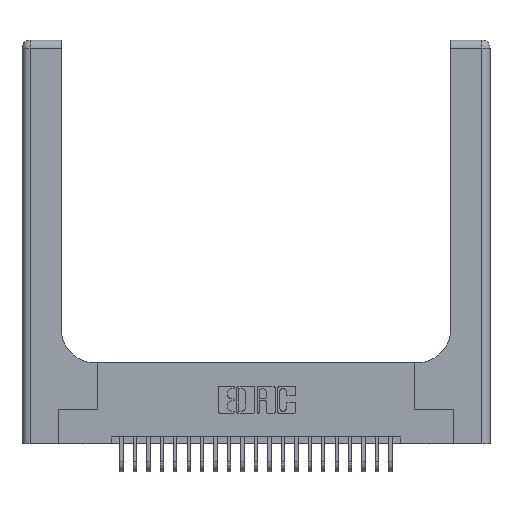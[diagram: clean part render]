
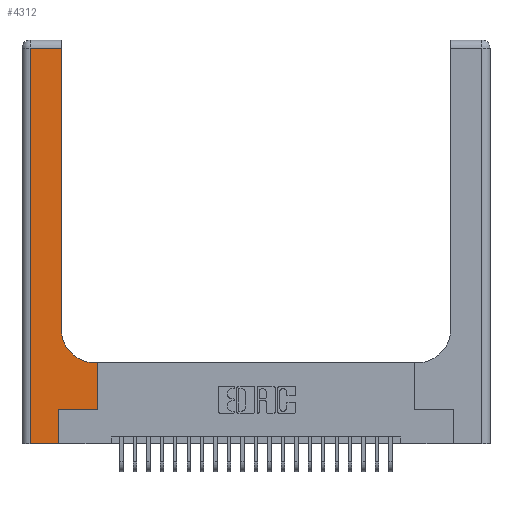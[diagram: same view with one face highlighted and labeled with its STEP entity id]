
A CAD part, top view. The second image highlights one B-rep face of the part: STEP entity #4312.
In plain terms, the highlighted planar face has unit normal (0, 0, 1).
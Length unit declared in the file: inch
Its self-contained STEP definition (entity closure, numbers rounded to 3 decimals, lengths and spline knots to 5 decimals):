
#283 = EDGE_CURVE ( 'NONE', #5069, #25096, #24114, .T. ) ;
#323 = EDGE_CURVE ( 'NONE', #25096, #14885, #16955, .T. ) ;
#327 = EDGE_CURVE ( 'NONE', #7880, #5069, #632, .T. ) ;
#428 = PLANE ( 'NONE',  #16071 ) ;
#632 = LINE ( 'NONE', #15826, #6159 ) ;
#633 = VECTOR ( 'NONE', #2783, 39.37008 ) ;
#689 = CARTESIAN_POINT ( 'NONE',  ( 0.2915, 3., 0.37 ) ) ;
#990 = EDGE_CURVE ( 'NONE', #6006, #20870, #8353, .T. ) ;
#1813 = EDGE_CURVE ( 'NONE', #12236, #6006, #19679, .T. ) ;
#1862 = CARTESIAN_POINT ( 'NONE',  ( 0.269, 0., 0.37 ) ) ;
#2422 = DIRECTION ( 'NONE',  ( 0., -1., 0. ) ) ;
#2451 = CARTESIAN_POINT ( 'NONE',  ( 0.06, 3., 0.37 ) ) ;
#2518 = DIRECTION ( 'NONE',  ( -1., 0., 0. ) ) ;
#2783 = DIRECTION ( 'NONE',  ( 0., 1., 0. ) ) ;
#3163 = ORIENTED_EDGE ( 'NONE', *, *, #327, .T. ) ;
#3535 = VECTOR ( 'NONE', #2422, 39.37008 ) ;
#3929 = CARTESIAN_POINT ( 'NONE',  ( 0.269, 0.25, 0.37 ) ) ;
#4312 = ADVANCED_FACE ( 'NONE', ( #22707 ), #428, .F. ) ;
#4832 = CARTESIAN_POINT ( 'NONE',  ( 0., 0., 0.37 ) ) ;
#5069 = VERTEX_POINT ( 'NONE', #22783 ) ;
#5085 = VECTOR ( 'NONE', #15970, 39.37008 ) ;
#6006 = VERTEX_POINT ( 'NONE', #21691 ) ;
#6017 = ORIENTED_EDGE ( 'NONE', *, *, #13298, .T. ) ;
#6159 = VECTOR ( 'NONE', #15813, 39.37008 ) ;
#6160 = LINE ( 'NONE', #689, #633 ) ;
#7880 = VERTEX_POINT ( 'NONE', #3929 ) ;
#7888 = CARTESIAN_POINT ( 'NONE',  ( 0.5585, 0.6, 0.37 ) ) ;
#8353 = LINE ( 'NONE', #2451, #3535 ) ;
#8730 = ORIENTED_EDGE ( 'NONE', *, *, #12244, .T. ) ;
#9877 = CARTESIAN_POINT ( 'NONE',  ( 0.2915, 2.94, 0.37 ) ) ;
#10706 = VECTOR ( 'NONE', #19007, 39.37008 ) ;
#11615 = VECTOR ( 'NONE', #16193, 39.37008 ) ;
#12059 = CARTESIAN_POINT ( 'NONE',  ( 0.5415, 0.85, 0.37 ) ) ;
#12167 = CIRCLE ( 'NONE', #18503, 0.25 ) ;
#12199 = EDGE_LOOP ( 'NONE', ( #18873, #17325, #25701, #20301, #6017, #3163, #23584, #18331, #8730 ) ) ;
#12236 = VERTEX_POINT ( 'NONE', #9877 ) ;
#12244 = EDGE_CURVE ( 'NONE', #14885, #24378, #12167, .T. ) ;
#12736 = CARTESIAN_POINT ( 'NONE',  ( 0.06, 0., 0.37 ) ) ;
#13298 = EDGE_CURVE ( 'NONE', #22804, #7880, #21219, .T. ) ;
#13933 = CARTESIAN_POINT ( 'NONE',  ( 0.269, 0., 0.37 ) ) ;
#14072 = DIRECTION ( 'NONE',  ( 1., 0., 0. ) ) ;
#14311 = DIRECTION ( 'NONE',  ( -1., 0., 0. ) ) ;
#14468 = CARTESIAN_POINT ( 'NONE',  ( 0., 2.94, 0.37 ) ) ;
#14797 = DIRECTION ( 'NONE',  ( 0., 0., -1. ) ) ;
#14885 = VERTEX_POINT ( 'NONE', #17413 ) ;
#15813 = DIRECTION ( 'NONE',  ( 1., 0., 0. ) ) ;
#15826 = CARTESIAN_POINT ( 'NONE',  ( 0.269, 0.25, 0.37 ) ) ;
#15970 = DIRECTION ( 'NONE',  ( 0., 1., 0. ) ) ;
#16071 = AXIS2_PLACEMENT_3D ( 'NONE', #22719, #14797, #2518 ) ;
#16088 = LINE ( 'NONE', #4832, #10706 ) ;
#16193 = DIRECTION ( 'NONE',  ( -1., 0., 0. ) ) ;
#16388 = EDGE_CURVE ( 'NONE', #20870, #22804, #16088, .T. ) ;
#16528 = CARTESIAN_POINT ( 'NONE',  ( 0.2915, 0.6, 0.37 ) ) ;
#16955 = LINE ( 'NONE', #16528, #11615 ) ;
#17131 = DIRECTION ( 'NONE',  ( 0., 1., 0. ) ) ;
#17325 = ORIENTED_EDGE ( 'NONE', *, *, #1813, .T. ) ;
#17413 = CARTESIAN_POINT ( 'NONE',  ( 0.5415, 0.6, 0.37 ) ) ;
#17574 = EDGE_CURVE ( 'NONE', #24378, #12236, #6160, .T. ) ;
#17821 = CARTESIAN_POINT ( 'NONE',  ( 0.5585, 0.25, 0.37 ) ) ;
#18204 = VECTOR ( 'NONE', #17131, 39.37008 ) ;
#18331 = ORIENTED_EDGE ( 'NONE', *, *, #323, .T. ) ;
#18503 = AXIS2_PLACEMENT_3D ( 'NONE', #12059, #25951, #14072 ) ;
#18873 = ORIENTED_EDGE ( 'NONE', *, *, #17574, .T. ) ;
#19007 = DIRECTION ( 'NONE',  ( 1., 0., 0. ) ) ;
#19050 = VECTOR ( 'NONE', #14311, 39.37008 ) ;
#19679 = LINE ( 'NONE', #14468, #19050 ) ;
#20301 = ORIENTED_EDGE ( 'NONE', *, *, #16388, .T. ) ;
#20870 = VERTEX_POINT ( 'NONE', #12736 ) ;
#21219 = LINE ( 'NONE', #13933, #5085 ) ;
#21691 = CARTESIAN_POINT ( 'NONE',  ( 0.06, 2.94, 0.37 ) ) ;
#22707 = FACE_OUTER_BOUND ( 'NONE', #12199, .T. ) ;
#22719 = CARTESIAN_POINT ( 'NONE',  ( 0., 3., 0.37 ) ) ;
#22783 = CARTESIAN_POINT ( 'NONE',  ( 0.5585, 0.25, 0.37 ) ) ;
#22804 = VERTEX_POINT ( 'NONE', #1862 ) ;
#23584 = ORIENTED_EDGE ( 'NONE', *, *, #283, .T. ) ;
#24114 = LINE ( 'NONE', #17821, #18204 ) ;
#24378 = VERTEX_POINT ( 'NONE', #25522 ) ;
#25096 = VERTEX_POINT ( 'NONE', #7888 ) ;
#25522 = CARTESIAN_POINT ( 'NONE',  ( 0.2915, 0.85, 0.37 ) ) ;
#25701 = ORIENTED_EDGE ( 'NONE', *, *, #990, .T. ) ;
#25951 = DIRECTION ( 'NONE',  ( 0., 0., -1. ) ) ;
